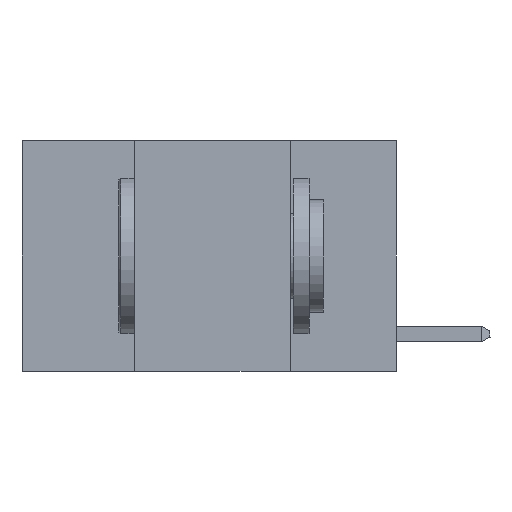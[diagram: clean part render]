
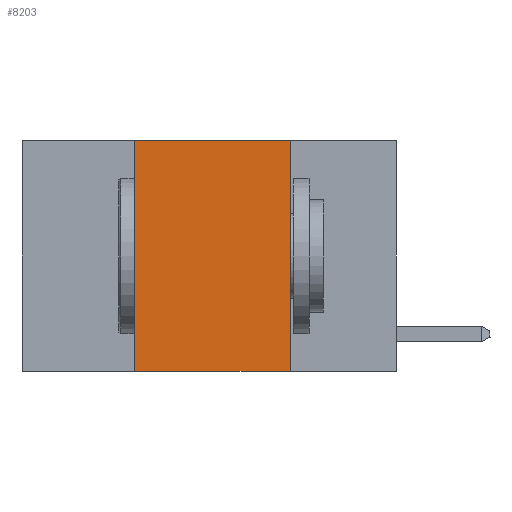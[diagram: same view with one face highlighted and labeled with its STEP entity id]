
A CAD part, left-side view. The second image highlights one B-rep face of the part: STEP entity #8203.
In plain terms, the highlighted planar face has unit normal (-1, 0, 0).
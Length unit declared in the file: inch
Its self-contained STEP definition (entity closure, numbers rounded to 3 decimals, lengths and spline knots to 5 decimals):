
#606 = VECTOR ( 'NONE', #9722, 39.37008 ) ;
#2208 = VERTEX_POINT ( 'NONE', #16788 ) ;
#2253 = VERTEX_POINT ( 'NONE', #3592 ) ;
#2285 = AXIS2_PLACEMENT_3D ( 'NONE', #6713, #10111, #21521 ) ;
#2644 = VERTEX_POINT ( 'NONE', #13021 ) ;
#3082 = LINE ( 'NONE', #4024, #20225 ) ;
#3442 = ORIENTED_EDGE ( 'NONE', *, *, #15743, .F. ) ;
#3592 = CARTESIAN_POINT ( 'NONE',  ( 0., 0.42, 0. ) ) ;
#4024 = CARTESIAN_POINT ( 'NONE',  ( 0., 0.42, 0. ) ) ;
#5117 = LINE ( 'NONE', #19548, #606 ) ;
#6713 = CARTESIAN_POINT ( 'NONE',  ( 0., 0.6, 0. ) ) ;
#6837 = VECTOR ( 'NONE', #14609, 39.37008 ) ;
#7082 = EDGE_CURVE ( 'NONE', #2208, #16755, #5117, .T. ) ;
#7361 = DIRECTION ( 'NONE',  ( 0., 0., 1. ) ) ;
#7464 = EDGE_LOOP ( 'NONE', ( #20053, #3442, #7933, #17246 ) ) ;
#7730 = CARTESIAN_POINT ( 'NONE',  ( 0., 0.6, 0. ) ) ;
#7933 = ORIENTED_EDGE ( 'NONE', *, *, #15608, .F. ) ;
#8203 = ADVANCED_FACE ( 'NONE', ( #19598 ), #13337, .F. ) ;
#9450 = LINE ( 'NONE', #7730, #9977 ) ;
#9601 = CARTESIAN_POINT ( 'NONE',  ( 0., 0.17, -0.37 ) ) ;
#9615 = CARTESIAN_POINT ( 'NONE',  ( 0., 0.17, 0. ) ) ;
#9722 = DIRECTION ( 'NONE',  ( 0., -1., 0. ) ) ;
#9977 = VECTOR ( 'NONE', #15954, 39.37008 ) ;
#10111 = DIRECTION ( 'NONE',  ( 1., 0., 0. ) ) ;
#13021 = CARTESIAN_POINT ( 'NONE',  ( 0., 0.17, 0. ) ) ;
#13337 = PLANE ( 'NONE',  #2285 ) ;
#14609 = DIRECTION ( 'NONE',  ( 0., 0., -1. ) ) ;
#15608 = EDGE_CURVE ( 'NONE', #2208, #2253, #3082, .T. ) ;
#15743 = EDGE_CURVE ( 'NONE', #2253, #2644, #9450, .T. ) ;
#15954 = DIRECTION ( 'NONE',  ( 0., -1., 0. ) ) ;
#16755 = VERTEX_POINT ( 'NONE', #9601 ) ;
#16788 = CARTESIAN_POINT ( 'NONE',  ( 0., 0.42, -0.37 ) ) ;
#17246 = ORIENTED_EDGE ( 'NONE', *, *, #7082, .T. ) ;
#19548 = CARTESIAN_POINT ( 'NONE',  ( 0., 0.6, -0.37 ) ) ;
#19598 = FACE_OUTER_BOUND ( 'NONE', #7464, .T. ) ;
#20018 = LINE ( 'NONE', #9615, #6837 ) ;
#20053 = ORIENTED_EDGE ( 'NONE', *, *, #21016, .F. ) ;
#20225 = VECTOR ( 'NONE', #7361, 39.37008 ) ;
#21016 = EDGE_CURVE ( 'NONE', #2644, #16755, #20018, .T. ) ;
#21521 = DIRECTION ( 'NONE',  ( 0., 0., -1. ) ) ;
